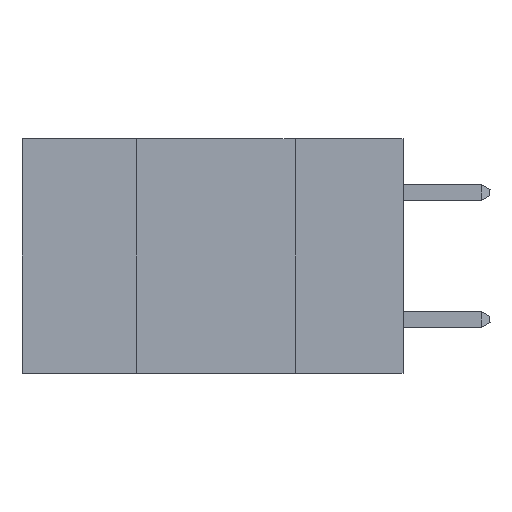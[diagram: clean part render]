
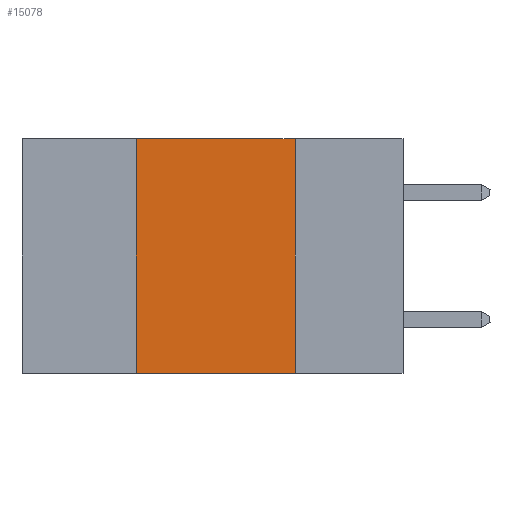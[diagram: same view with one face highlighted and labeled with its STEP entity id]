
A CAD part, left-side view. The second image highlights one B-rep face of the part: STEP entity #15078.
In plain terms, the highlighted planar face has unit normal (-1, 0, 0).
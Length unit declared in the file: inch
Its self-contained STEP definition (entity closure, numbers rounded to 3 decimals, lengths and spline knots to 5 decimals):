
#1298 = VECTOR ( 'NONE', #23169, 39.37008 ) ;
#1964 = LINE ( 'NONE', #1970, #1298 ) ;
#1970 = CARTESIAN_POINT ( 'NONE',  ( 0., 0.6, 0. ) ) ;
#2143 = EDGE_CURVE ( 'NONE', #24903, #21969, #10402, .T. ) ;
#2493 = LINE ( 'NONE', #20677, #18801 ) ;
#2643 = DIRECTION ( 'NONE',  ( 0., 0., -1. ) ) ;
#2815 = ORIENTED_EDGE ( 'NONE', *, *, #2143, .F. ) ;
#3231 = EDGE_CURVE ( 'NONE', #25806, #24769, #11654, .T. ) ;
#3505 = CARTESIAN_POINT ( 'NONE',  ( 0., 0.42, 0. ) ) ;
#6771 = CARTESIAN_POINT ( 'NONE',  ( 0., 0.17, -0.37 ) ) ;
#6939 = DIRECTION ( 'NONE',  ( 0., 0., -1. ) ) ;
#7807 = FACE_OUTER_BOUND ( 'NONE', #12538, .T. ) ;
#9343 = AXIS2_PLACEMENT_3D ( 'NONE', #15338, #15430, #2643 ) ;
#9369 = CARTESIAN_POINT ( 'NONE',  ( 0., 0.42, -0.37 ) ) ;
#10086 = EDGE_CURVE ( 'NONE', #25806, #21969, #2493, .T. ) ;
#10402 = LINE ( 'NONE', #26972, #20974 ) ;
#11654 = LINE ( 'NONE', #17654, #27026 ) ;
#12538 = EDGE_LOOP ( 'NONE', ( #2815, #13513, #20435, #25948 ) ) ;
#13513 = ORIENTED_EDGE ( 'NONE', *, *, #18957, .F. ) ;
#15078 = ADVANCED_FACE ( 'NONE', ( #7807 ), #21649, .F. ) ;
#15338 = CARTESIAN_POINT ( 'NONE',  ( 0., 0.6, 0. ) ) ;
#15430 = DIRECTION ( 'NONE',  ( 1., 0., 0. ) ) ;
#17261 = DIRECTION ( 'NONE',  ( 0., 0., 1. ) ) ;
#17654 = CARTESIAN_POINT ( 'NONE',  ( 0., 0.42, 0. ) ) ;
#18801 = VECTOR ( 'NONE', #24866, 39.37008 ) ;
#18957 = EDGE_CURVE ( 'NONE', #24769, #24903, #1964, .T. ) ;
#20435 = ORIENTED_EDGE ( 'NONE', *, *, #3231, .F. ) ;
#20677 = CARTESIAN_POINT ( 'NONE',  ( 0., 0.6, -0.37 ) ) ;
#20854 = CARTESIAN_POINT ( 'NONE',  ( 0., 0.17, 0. ) ) ;
#20974 = VECTOR ( 'NONE', #6939, 39.37008 ) ;
#21649 = PLANE ( 'NONE',  #9343 ) ;
#21969 = VERTEX_POINT ( 'NONE', #6771 ) ;
#23169 = DIRECTION ( 'NONE',  ( 0., -1., 0. ) ) ;
#24769 = VERTEX_POINT ( 'NONE', #3505 ) ;
#24866 = DIRECTION ( 'NONE',  ( 0., -1., 0. ) ) ;
#24903 = VERTEX_POINT ( 'NONE', #20854 ) ;
#25806 = VERTEX_POINT ( 'NONE', #9369 ) ;
#25948 = ORIENTED_EDGE ( 'NONE', *, *, #10086, .T. ) ;
#26972 = CARTESIAN_POINT ( 'NONE',  ( 0., 0.17, 0. ) ) ;
#27026 = VECTOR ( 'NONE', #17261, 39.37008 ) ;
